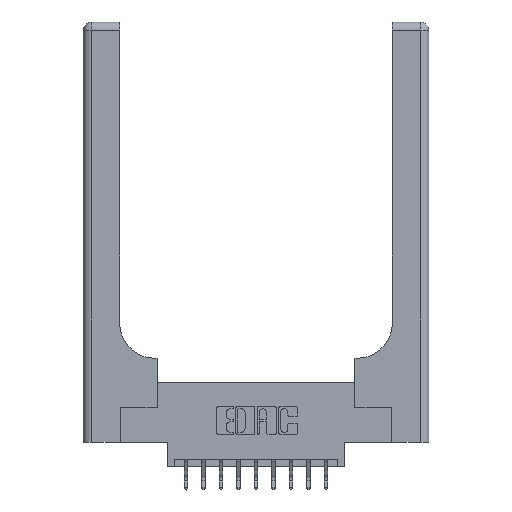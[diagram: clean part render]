
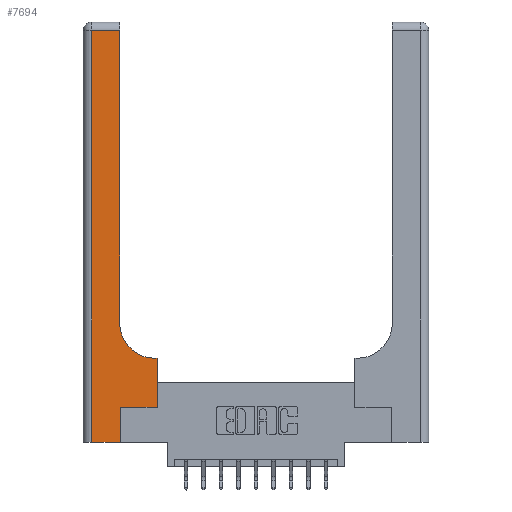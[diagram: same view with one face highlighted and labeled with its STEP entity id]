
A CAD part, top view. The second image highlights one B-rep face of the part: STEP entity #7694.
In plain terms, the highlighted planar face has unit normal (0, 0, 1).
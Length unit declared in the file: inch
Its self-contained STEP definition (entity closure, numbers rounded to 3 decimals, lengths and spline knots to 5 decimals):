
#4 = CARTESIAN_POINT ( 'NONE',  ( 0.265, 0.25, 0.37 ) ) ;
#48 = DIRECTION ( 'NONE',  ( 1., 0., 0. ) ) ;
#168 = ORIENTED_EDGE ( 'NONE', *, *, #14133, .T. ) ;
#220 = VECTOR ( 'NONE', #3408, 39.37008 ) ;
#757 = CIRCLE ( 'NONE', #7286, 0.25 ) ;
#817 = VECTOR ( 'NONE', #10081, 39.37008 ) ;
#826 = EDGE_CURVE ( 'NONE', #4091, #11682, #15653, .T. ) ;
#985 = CARTESIAN_POINT ( 'NONE',  ( 0.26, 3., 0.37 ) ) ;
#1932 = VERTEX_POINT ( 'NONE', #9971 ) ;
#2048 = DIRECTION ( 'NONE',  ( -1., 0., 0. ) ) ;
#2152 = VERTEX_POINT ( 'NONE', #11547 ) ;
#2221 = CARTESIAN_POINT ( 'NONE',  ( 0.265, 0., 0.37 ) ) ;
#2302 = VECTOR ( 'NONE', #2048, 39.37008 ) ;
#2508 = CARTESIAN_POINT ( 'NONE',  ( 0.265, 0.25, 0.37 ) ) ;
#2708 = VECTOR ( 'NONE', #48, 39.37008 ) ;
#2775 = ORIENTED_EDGE ( 'NONE', *, *, #4235, .T. ) ;
#3016 = LINE ( 'NONE', #4782, #12340 ) ;
#3408 = DIRECTION ( 'NONE',  ( 1., 0., 0. ) ) ;
#3421 = CARTESIAN_POINT ( 'NONE',  ( 0.51, 0.85, 0.37 ) ) ;
#3449 = DIRECTION ( 'NONE',  ( 0., 1., 0. ) ) ;
#3541 = LINE ( 'NONE', #8259, #220 ) ;
#4091 = VERTEX_POINT ( 'NONE', #2508 ) ;
#4137 = LINE ( 'NONE', #13696, #817 ) ;
#4235 = EDGE_CURVE ( 'NONE', #13055, #2152, #4137, .T. ) ;
#4643 = DIRECTION ( 'NONE',  ( 1., 0., 0. ) ) ;
#4703 = LINE ( 'NONE', #9891, #11177 ) ;
#4734 = PLANE ( 'NONE',  #13195 ) ;
#4782 = CARTESIAN_POINT ( 'NONE',  ( 0.06, 3., 0.37 ) ) ;
#4919 = VECTOR ( 'NONE', #3449, 39.37008 ) ;
#5751 = EDGE_CURVE ( 'NONE', #12287, #8530, #3541, .T. ) ;
#6581 = ORIENTED_EDGE ( 'NONE', *, *, #9877, .T. ) ;
#7012 = EDGE_CURVE ( 'NONE', #9809, #14050, #757, .T. ) ;
#7193 = DIRECTION ( 'NONE',  ( -1., 0., 0. ) ) ;
#7286 = AXIS2_PLACEMENT_3D ( 'NONE', #3421, #11937, #4643 ) ;
#7668 = VECTOR ( 'NONE', #15625, 39.37008 ) ;
#7694 = ADVANCED_FACE ( 'NONE', ( #13148 ), #4734, .F. ) ;
#7729 = ORIENTED_EDGE ( 'NONE', *, *, #5751, .T. ) ;
#8141 = CARTESIAN_POINT ( 'NONE',  ( 0.26, 0.85, 0.37 ) ) ;
#8259 = CARTESIAN_POINT ( 'NONE',  ( 0., 0., 0.37 ) ) ;
#8354 = CARTESIAN_POINT ( 'NONE',  ( 0.51, 0.6, 0.37 ) ) ;
#8530 = VERTEX_POINT ( 'NONE', #8773 ) ;
#8773 = CARTESIAN_POINT ( 'NONE',  ( 0.265, 0., 0.37 ) ) ;
#9101 = CARTESIAN_POINT ( 'NONE',  ( 0.528, 0.25, 0.37 ) ) ;
#9310 = EDGE_LOOP ( 'NONE', ( #168, #2775, #6581, #7729, #10073, #12335, #13483, #11240, #10658 ) ) ;
#9797 = EDGE_CURVE ( 'NONE', #8530, #4091, #13875, .T. ) ;
#9809 = VERTEX_POINT ( 'NONE', #8354 ) ;
#9877 = EDGE_CURVE ( 'NONE', #2152, #12287, #3016, .T. ) ;
#9891 = CARTESIAN_POINT ( 'NONE',  ( 0.528, 0.25, 0.37 ) ) ;
#9971 = CARTESIAN_POINT ( 'NONE',  ( 0.528, 0.6, 0.37 ) ) ;
#10073 = ORIENTED_EDGE ( 'NONE', *, *, #9797, .T. ) ;
#10081 = DIRECTION ( 'NONE',  ( -1., 0., 0. ) ) ;
#10463 = EDGE_CURVE ( 'NONE', #11682, #1932, #4703, .T. ) ;
#10580 = CARTESIAN_POINT ( 'NONE',  ( 0.26, 0.6, 0.37 ) ) ;
#10658 = ORIENTED_EDGE ( 'NONE', *, *, #7012, .T. ) ;
#10895 = DIRECTION ( 'NONE',  ( 0., -1., 0. ) ) ;
#11086 = DIRECTION ( 'NONE',  ( 0., 1., 0. ) ) ;
#11177 = VECTOR ( 'NONE', #11086, 39.37008 ) ;
#11191 = CARTESIAN_POINT ( 'NONE',  ( 0.26, 2.94, 0.37 ) ) ;
#11240 = ORIENTED_EDGE ( 'NONE', *, *, #14047, .T. ) ;
#11255 = LINE ( 'NONE', #985, #7668 ) ;
#11547 = CARTESIAN_POINT ( 'NONE',  ( 0.06, 2.94, 0.37 ) ) ;
#11682 = VERTEX_POINT ( 'NONE', #9101 ) ;
#11937 = DIRECTION ( 'NONE',  ( 0., 0., -1. ) ) ;
#12287 = VERTEX_POINT ( 'NONE', #15411 ) ;
#12335 = ORIENTED_EDGE ( 'NONE', *, *, #826, .T. ) ;
#12340 = VECTOR ( 'NONE', #10895, 39.37008 ) ;
#13055 = VERTEX_POINT ( 'NONE', #11191 ) ;
#13148 = FACE_OUTER_BOUND ( 'NONE', #9310, .T. ) ;
#13195 = AXIS2_PLACEMENT_3D ( 'NONE', #13254, #14474, #7193 ) ;
#13254 = CARTESIAN_POINT ( 'NONE',  ( 0., 3., 0.37 ) ) ;
#13483 = ORIENTED_EDGE ( 'NONE', *, *, #10463, .T. ) ;
#13696 = CARTESIAN_POINT ( 'NONE',  ( 0., 2.94, 0.37 ) ) ;
#13875 = LINE ( 'NONE', #2221, #4919 ) ;
#14047 = EDGE_CURVE ( 'NONE', #1932, #9809, #14890, .T. ) ;
#14050 = VERTEX_POINT ( 'NONE', #8141 ) ;
#14133 = EDGE_CURVE ( 'NONE', #14050, #13055, #11255, .T. ) ;
#14474 = DIRECTION ( 'NONE',  ( 0., 0., -1. ) ) ;
#14890 = LINE ( 'NONE', #10580, #2302 ) ;
#15411 = CARTESIAN_POINT ( 'NONE',  ( 0.06, 0., 0.37 ) ) ;
#15625 = DIRECTION ( 'NONE',  ( 0., 1., 0. ) ) ;
#15653 = LINE ( 'NONE', #4, #2708 ) ;
